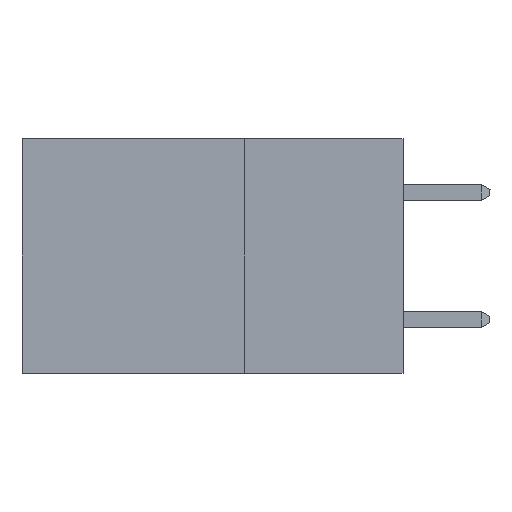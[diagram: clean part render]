
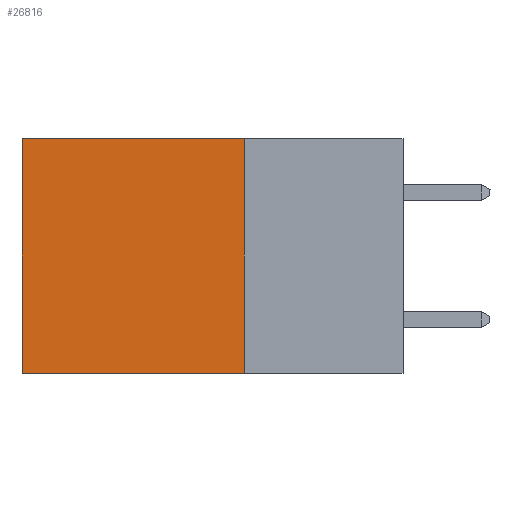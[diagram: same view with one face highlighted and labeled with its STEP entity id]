
A CAD part, left-side view. The second image highlights one B-rep face of the part: STEP entity #26816.
In plain terms, the highlighted planar face has unit normal (-1, 0, 0).
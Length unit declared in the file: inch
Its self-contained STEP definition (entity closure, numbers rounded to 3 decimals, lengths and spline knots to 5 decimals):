
#702 = CARTESIAN_POINT ( 'NONE',  ( 0.2875, 0.25, -0.37 ) ) ;
#2574 = LINE ( 'NONE', #32754, #9398 ) ;
#3964 = EDGE_LOOP ( 'NONE', ( #32522, #8960, #28256, #37290 ) ) ;
#4224 = VERTEX_POINT ( 'NONE', #15791 ) ;
#4432 = CARTESIAN_POINT ( 'NONE',  ( 0.2875, 0.25, 0. ) ) ;
#7794 = DIRECTION ( 'NONE',  ( 1., 0., 0. ) ) ;
#8960 = ORIENTED_EDGE ( 'NONE', *, *, #27811, .F. ) ;
#9096 = DIRECTION ( 'NONE',  ( 0., 0., -1. ) ) ;
#9398 = VECTOR ( 'NONE', #29594, 39.37008 ) ;
#11161 = VECTOR ( 'NONE', #42751, 39.37008 ) ;
#12046 = VERTEX_POINT ( 'NONE', #29977 ) ;
#12080 = VECTOR ( 'NONE', #30464, 39.37008 ) ;
#12171 = FACE_OUTER_BOUND ( 'NONE', #3964, .T. ) ;
#15791 = CARTESIAN_POINT ( 'NONE',  ( 0.2875, 0.6, 0. ) ) ;
#20869 = VERTEX_POINT ( 'NONE', #27343 ) ;
#21478 = EDGE_CURVE ( 'NONE', #20869, #4224, #29928, .T. ) ;
#25709 = VECTOR ( 'NONE', #9096, 39.37008 ) ;
#26816 = ADVANCED_FACE ( 'NONE', ( #12171 ), #27940, .F. ) ;
#27153 = CARTESIAN_POINT ( 'NONE',  ( 0.2875, 0.25, 0. ) ) ;
#27343 = CARTESIAN_POINT ( 'NONE',  ( 0.2875, 0.25, 0. ) ) ;
#27811 = EDGE_CURVE ( 'NONE', #38202, #12046, #37799, .T. ) ;
#27940 = PLANE ( 'NONE',  #36119 ) ;
#28256 = ORIENTED_EDGE ( 'NONE', *, *, #35204, .F. ) ;
#29594 = DIRECTION ( 'NONE',  ( 0., 0., -1. ) ) ;
#29928 = LINE ( 'NONE', #27153, #12080 ) ;
#29977 = CARTESIAN_POINT ( 'NONE',  ( 0.2875, 0.6, -0.37 ) ) ;
#30464 = DIRECTION ( 'NONE',  ( 0., 1., 0. ) ) ;
#31237 = DIRECTION ( 'NONE',  ( 0., 0., -1. ) ) ;
#32522 = ORIENTED_EDGE ( 'NONE', *, *, #34555, .T. ) ;
#32533 = CARTESIAN_POINT ( 'NONE',  ( 0.2875, 0.25, 0. ) ) ;
#32754 = CARTESIAN_POINT ( 'NONE',  ( 0.2875, 0.6, 0. ) ) ;
#34555 = EDGE_CURVE ( 'NONE', #4224, #12046, #2574, .T. ) ;
#35204 = EDGE_CURVE ( 'NONE', #20869, #38202, #43272, .T. ) ;
#36119 = AXIS2_PLACEMENT_3D ( 'NONE', #4432, #7794, #31237 ) ;
#37290 = ORIENTED_EDGE ( 'NONE', *, *, #21478, .T. ) ;
#37799 = LINE ( 'NONE', #39409, #11161 ) ;
#38202 = VERTEX_POINT ( 'NONE', #702 ) ;
#39409 = CARTESIAN_POINT ( 'NONE',  ( 0.2875, 0.25, -0.37 ) ) ;
#42751 = DIRECTION ( 'NONE',  ( 0., 1., 0. ) ) ;
#43272 = LINE ( 'NONE', #32533, #25709 ) ;
